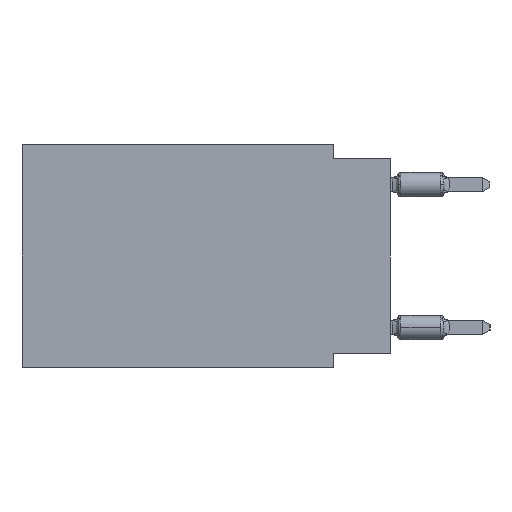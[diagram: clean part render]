
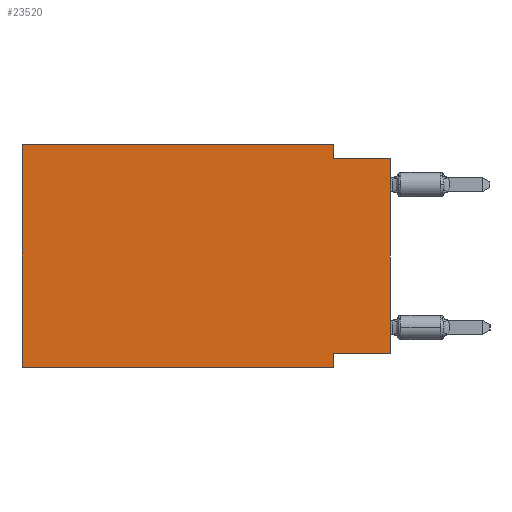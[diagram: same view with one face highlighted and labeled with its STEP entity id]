
A CAD part, left-side view. The second image highlights one B-rep face of the part: STEP entity #23520.
In plain terms, the highlighted planar face has unit normal (-1, 0, 0).
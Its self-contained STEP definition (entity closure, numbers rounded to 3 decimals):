
#453 = DIRECTION ( 'NONE',  ( 0., 0., 1. ) ) ;
#707 = VERTEX_POINT ( 'NONE', #26435 ) ;
#1449 = VERTEX_POINT ( 'NONE', #15638 ) ;
#1901 = VERTEX_POINT ( 'NONE', #15452 ) ;
#2031 = DIRECTION ( 'NONE',  ( 0., -1., 0. ) ) ;
#2176 = LINE ( 'NONE', #17501, #14627 ) ;
#2181 = DIRECTION ( 'NONE',  ( 0., 1., 0. ) ) ;
#2801 = LINE ( 'NONE', #9099, #8408 ) ;
#2888 = PLANE ( 'NONE',  #17588 ) ;
#3523 = EDGE_CURVE ( 'NONE', #5140, #9278, #24047, .T. ) ;
#3986 = ORIENTED_EDGE ( 'NONE', *, *, #26697, .T. ) ;
#4058 = VERTEX_POINT ( 'NONE', #22436 ) ;
#4313 = CARTESIAN_POINT ( 'NONE',  ( 0., 16.383, -9.906 ) ) ;
#4400 = CARTESIAN_POINT ( 'NONE',  ( 0., 0., -0.635 ) ) ;
#4467 = CARTESIAN_POINT ( 'NONE',  ( 0., 16.383, 0. ) ) ;
#4606 = DIRECTION ( 'NONE',  ( 0., -1., 0. ) ) ;
#4884 = LINE ( 'NONE', #7178, #26438 ) ;
#5140 = VERTEX_POINT ( 'NONE', #26634 ) ;
#6090 = EDGE_CURVE ( 'NONE', #14364, #5140, #4884, .T. ) ;
#6914 = LINE ( 'NONE', #4467, #19114 ) ;
#7178 = CARTESIAN_POINT ( 'NONE',  ( 0., 2.54, 0. ) ) ;
#8408 = VECTOR ( 'NONE', #9532, 1000. ) ;
#8414 = EDGE_CURVE ( 'NONE', #1449, #4058, #6914, .T. ) ;
#9099 = CARTESIAN_POINT ( 'NONE',  ( 0., 2.54, -9.906 ) ) ;
#9278 = VERTEX_POINT ( 'NONE', #21030 ) ;
#9532 = DIRECTION ( 'NONE',  ( 0., 0., -1. ) ) ;
#10793 = VECTOR ( 'NONE', #13132, 1000. ) ;
#11446 = ORIENTED_EDGE ( 'NONE', *, *, #22587, .F. ) ;
#11450 = ORIENTED_EDGE ( 'NONE', *, *, #3523, .F. ) ;
#11641 = DIRECTION ( 'NONE',  ( 1., 0., 0. ) ) ;
#11923 = CARTESIAN_POINT ( 'NONE',  ( 0., 16.383, 0. ) ) ;
#13132 = DIRECTION ( 'NONE',  ( 0., -1., 0. ) ) ;
#13236 = VECTOR ( 'NONE', #19383, 1000. ) ;
#14193 = FACE_OUTER_BOUND ( 'NONE', #17718, .T. ) ;
#14349 = EDGE_CURVE ( 'NONE', #1449, #1901, #24251, .T. ) ;
#14364 = VERTEX_POINT ( 'NONE', #24099 ) ;
#14627 = VECTOR ( 'NONE', #2031, 1000. ) ;
#14900 = CARTESIAN_POINT ( 'NONE',  ( 0., 2.54, -9.271 ) ) ;
#15220 = LINE ( 'NONE', #23987, #26064 ) ;
#15452 = CARTESIAN_POINT ( 'NONE',  ( 0., 2.54, -9.906 ) ) ;
#15638 = CARTESIAN_POINT ( 'NONE',  ( 0., 16.383, -9.906 ) ) ;
#16146 = ORIENTED_EDGE ( 'NONE', *, *, #6090, .F. ) ;
#16426 = ORIENTED_EDGE ( 'NONE', *, *, #8414, .F. ) ;
#16631 = ORIENTED_EDGE ( 'NONE', *, *, #26416, .F. ) ;
#17501 = CARTESIAN_POINT ( 'NONE',  ( 0., 16.383, 0. ) ) ;
#17588 = AXIS2_PLACEMENT_3D ( 'NONE', #11923, #11641, #27276 ) ;
#17718 = EDGE_LOOP ( 'NONE', ( #3986, #11450, #16146, #11446, #16426, #18305, #16631, #24277 ) ) ;
#18305 = ORIENTED_EDGE ( 'NONE', *, *, #14349, .T. ) ;
#18356 = VECTOR ( 'NONE', #4606, 1000. ) ;
#19114 = VECTOR ( 'NONE', #453, 1000. ) ;
#19246 = CARTESIAN_POINT ( 'NONE',  ( 0., 0., 0. ) ) ;
#19383 = DIRECTION ( 'NONE',  ( 0., 0., 1. ) ) ;
#21030 = CARTESIAN_POINT ( 'NONE',  ( 0., 0., -0.635 ) ) ;
#22436 = CARTESIAN_POINT ( 'NONE',  ( 0., 16.383, 0. ) ) ;
#22587 = EDGE_CURVE ( 'NONE', #4058, #14364, #2176, .T. ) ;
#23520 = ADVANCED_FACE ( 'NONE', ( #14193 ), #2888, .F. ) ;
#23987 = CARTESIAN_POINT ( 'NONE',  ( 0., 0., -9.271 ) ) ;
#24047 = LINE ( 'NONE', #4400, #10793 ) ;
#24099 = CARTESIAN_POINT ( 'NONE',  ( 0., 2.54, 0. ) ) ;
#24251 = LINE ( 'NONE', #4313, #18356 ) ;
#24277 = ORIENTED_EDGE ( 'NONE', *, *, #26754, .F. ) ;
#26064 = VECTOR ( 'NONE', #2181, 1000. ) ;
#26148 = LINE ( 'NONE', #19246, #13236 ) ;
#26416 = EDGE_CURVE ( 'NONE', #28255, #1901, #2801, .T. ) ;
#26435 = CARTESIAN_POINT ( 'NONE',  ( 0., 0., -9.271 ) ) ;
#26438 = VECTOR ( 'NONE', #26995, 1000. ) ;
#26634 = CARTESIAN_POINT ( 'NONE',  ( 0., 2.54, -0.635 ) ) ;
#26697 = EDGE_CURVE ( 'NONE', #707, #9278, #26148, .T. ) ;
#26754 = EDGE_CURVE ( 'NONE', #707, #28255, #15220, .T. ) ;
#26995 = DIRECTION ( 'NONE',  ( 0., 0., -1. ) ) ;
#27276 = DIRECTION ( 'NONE',  ( 0., 0., -1. ) ) ;
#28255 = VERTEX_POINT ( 'NONE', #14900 ) ;
